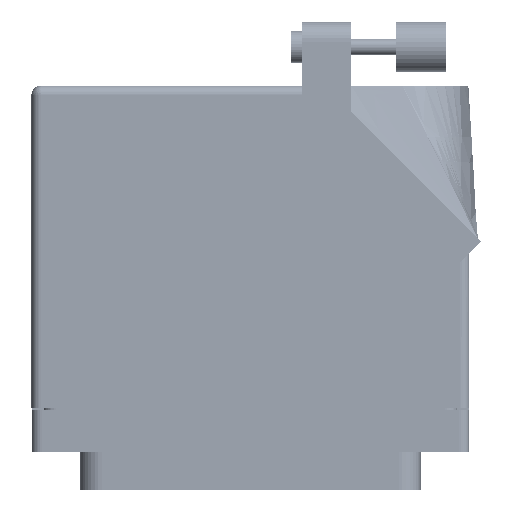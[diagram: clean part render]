
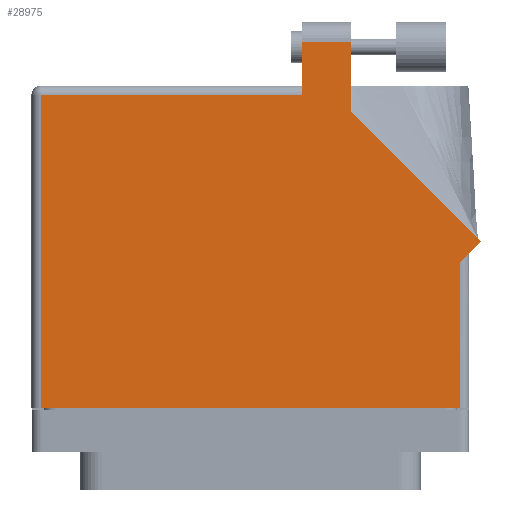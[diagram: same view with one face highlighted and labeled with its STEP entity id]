
A CAD part, front view. The second image highlights one B-rep face of the part: STEP entity #28975.
In plain terms, the highlighted face is planar.
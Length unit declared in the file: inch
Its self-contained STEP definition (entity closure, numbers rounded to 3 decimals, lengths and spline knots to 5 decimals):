
#886 = CARTESIAN_POINT ( 'NONE',  ( 1.3155, 0.88, 0.765 ) ) ;
#3059 = VECTOR ( 'NONE', #84220, 39.37008 ) ;
#3594 = CARTESIAN_POINT ( 'NONE',  ( 0.3275, 2.205, 0.765 ) ) ;
#3765 = VERTEX_POINT ( 'NONE', #63926 ) ;
#4632 = DIRECTION ( 'NONE',  ( 0., 1., 0. ) ) ;
#4713 = VECTOR ( 'NONE', #52360, 39.37008 ) ;
#5419 = LINE ( 'NONE', #886, #51687 ) ;
#9876 = VERTEX_POINT ( 'NONE', #50073 ) ;
#15484 = EDGE_CURVE ( 'NONE', #55758, #40353, #31630, .T. ) ;
#16427 = VECTOR ( 'NONE', #69184, 39.37008 ) ;
#19889 = CARTESIAN_POINT ( 'NONE',  ( 0.6345, 2.205, 0.765 ) ) ;
#20961 = AXIS2_PLACEMENT_3D ( 'NONE', #44829, #78649, #31268 ) ;
#22364 = EDGE_CURVE ( 'NONE', #66948, #9876, #5419, .T. ) ;
#22508 = VERTEX_POINT ( 'NONE', #69041 ) ;
#24976 = DIRECTION ( 'NONE',  ( 1., 0., 0. ) ) ;
#25692 = CARTESIAN_POINT ( 'NONE',  ( -1.3155, -0.1, 0.765 ) ) ;
#26282 = ORIENTED_EDGE ( 'NONE', *, *, #71351, .T. ) ;
#28975 = ADVANCED_FACE ( 'NONE', ( #63953 ), #58068, .F. ) ;
#31268 = DIRECTION ( 'NONE',  ( -1., 0., 0. ) ) ;
#31630 = LINE ( 'NONE', #3594, #4713 ) ;
#31757 = ORIENTED_EDGE ( 'NONE', *, *, #50247, .T. ) ;
#34848 = DIRECTION ( 'NONE',  ( 0., 1., 0. ) ) ;
#34971 = ORIENTED_EDGE ( 'NONE', *, *, #49040, .T. ) ;
#36153 = ORIENTED_EDGE ( 'NONE', *, *, #22364, .T. ) ;
#38192 = ORIENTED_EDGE ( 'NONE', *, *, #48228, .T. ) ;
#39518 = ORIENTED_EDGE ( 'NONE', *, *, #78637, .T. ) ;
#40353 = VERTEX_POINT ( 'NONE', #51179 ) ;
#41820 = LINE ( 'NONE', #50671, #3059 ) ;
#44149 = VECTOR ( 'NONE', #70210, 39.37008 ) ;
#44829 = CARTESIAN_POINT ( 'NONE',  ( -1.3775, 1.93, 0.765 ) ) ;
#45401 = CARTESIAN_POINT ( 'NONE',  ( 0.3275, 1.868, 0.765 ) ) ;
#46209 = LINE ( 'NONE', #72720, #60210 ) ;
#46398 = CARTESIAN_POINT ( 'NONE',  ( 1.44821, 0.95071, 0.765 ) ) ;
#47530 = VECTOR ( 'NONE', #64934, 39.37008 ) ;
#48228 = EDGE_CURVE ( 'NONE', #56273, #22508, #78715, .T. ) ;
#48633 = LINE ( 'NONE', #85797, #47530 ) ;
#49040 = EDGE_CURVE ( 'NONE', #22508, #55758, #46209, .T. ) ;
#49596 = LINE ( 'NONE', #65840, #70180 ) ;
#50073 = CARTESIAN_POINT ( 'NONE',  ( 1.3155, 0.818, 0.765 ) ) ;
#50199 = LINE ( 'NONE', #52403, #83736 ) ;
#50247 = EDGE_CURVE ( 'NONE', #9876, #56273, #41820, .T. ) ;
#50671 = CARTESIAN_POINT ( 'NONE',  ( 1.3775, 0.88, 0.765 ) ) ;
#51179 = CARTESIAN_POINT ( 'NONE',  ( 0.3275, 2.205, 0.765 ) ) ;
#51687 = VECTOR ( 'NONE', #34848, 39.37008 ) ;
#52360 = DIRECTION ( 'NONE',  ( -1., 0., 0. ) ) ;
#52403 = CARTESIAN_POINT ( 'NONE',  ( -1.3775, -0.1, 0.765 ) ) ;
#53012 = LINE ( 'NONE', #54658, #16427 ) ;
#54106 = EDGE_LOOP ( 'NONE', ( #34971, #82132, #61737, #39518, #26282, #86371, #36153, #31757, #38192 ) ) ;
#54658 = CARTESIAN_POINT ( 'NONE',  ( -1.3155, -0.1, 0.765 ) ) ;
#55758 = VERTEX_POINT ( 'NONE', #19889 ) ;
#56273 = VERTEX_POINT ( 'NONE', #46398 ) ;
#57883 = EDGE_CURVE ( 'NONE', #40353, #83420, #49596, .T. ) ;
#58068 = PLANE ( 'NONE',  #20961 ) ;
#60210 = VECTOR ( 'NONE', #4632, 39.37008 ) ;
#61737 = ORIENTED_EDGE ( 'NONE', *, *, #57883, .T. ) ;
#63236 = CARTESIAN_POINT ( 'NONE',  ( 1.3155, -0.1, 0.765 ) ) ;
#63851 = CARTESIAN_POINT ( 'NONE',  ( 1.44821, 0.95071, 0.765 ) ) ;
#63926 = CARTESIAN_POINT ( 'NONE',  ( -1.3155, 1.868, 0.765 ) ) ;
#63953 = FACE_OUTER_BOUND ( 'NONE', #54106, .T. ) ;
#64934 = DIRECTION ( 'NONE',  ( -1., 0., 0. ) ) ;
#65840 = CARTESIAN_POINT ( 'NONE',  ( 0.3275, 1.93, 0.765 ) ) ;
#66455 = DIRECTION ( 'NONE',  ( 0., -1., 0. ) ) ;
#66948 = VERTEX_POINT ( 'NONE', #63236 ) ;
#69041 = CARTESIAN_POINT ( 'NONE',  ( 0.6345, 1.76442, 0.765 ) ) ;
#69184 = DIRECTION ( 'NONE',  ( 0., -1., 0. ) ) ;
#70180 = VECTOR ( 'NONE', #66455, 39.37008 ) ;
#70210 = DIRECTION ( 'NONE',  ( -0.707, 0.707, 0. ) ) ;
#71351 = EDGE_CURVE ( 'NONE', #3765, #79637, #53012, .T. ) ;
#72720 = CARTESIAN_POINT ( 'NONE',  ( 0.6345, 1.76442, 0.765 ) ) ;
#78637 = EDGE_CURVE ( 'NONE', #83420, #3765, #48633, .T. ) ;
#78649 = DIRECTION ( 'NONE',  ( 0., 0., -1. ) ) ;
#78715 = LINE ( 'NONE', #63851, #44149 ) ;
#79637 = VERTEX_POINT ( 'NONE', #25692 ) ;
#82132 = ORIENTED_EDGE ( 'NONE', *, *, #15484, .T. ) ;
#83420 = VERTEX_POINT ( 'NONE', #45401 ) ;
#83736 = VECTOR ( 'NONE', #24976, 39.37008 ) ;
#84220 = DIRECTION ( 'NONE',  ( 0.707, 0.707, 0. ) ) ;
#84241 = EDGE_CURVE ( 'NONE', #79637, #66948, #50199, .T. ) ;
#85797 = CARTESIAN_POINT ( 'NONE',  ( -1.3775, 1.868, 0.765 ) ) ;
#86371 = ORIENTED_EDGE ( 'NONE', *, *, #84241, .T. ) ;
